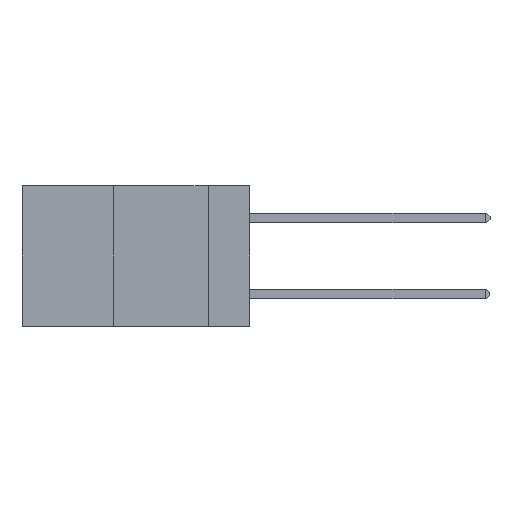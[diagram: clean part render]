
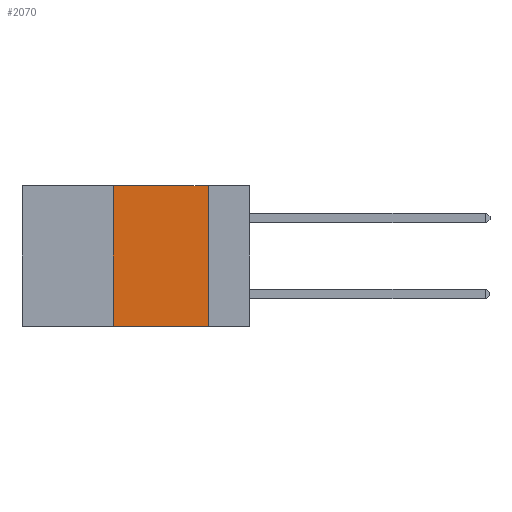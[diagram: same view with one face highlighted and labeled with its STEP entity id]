
A CAD part, left-side view. The second image highlights one B-rep face of the part: STEP entity #2070.
In plain terms, the highlighted planar face has unit normal (-1, 0, 0).
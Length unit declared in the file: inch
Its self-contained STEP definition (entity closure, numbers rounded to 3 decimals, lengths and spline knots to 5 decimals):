
#400 = VERTEX_POINT ( 'NONE', #1898 ) ;
#686 = CARTESIAN_POINT ( 'NONE',  ( 0., 0.36, 0. ) ) ;
#805 = LINE ( 'NONE', #8041, #7409 ) ;
#1435 = DIRECTION ( 'NONE',  ( 1., 0., 0. ) ) ;
#1520 = DIRECTION ( 'NONE',  ( 0., 0., -1. ) ) ;
#1556 = DIRECTION ( 'NONE',  ( 0., 0., 1. ) ) ;
#1810 = LINE ( 'NONE', #4463, #9916 ) ;
#1898 = CARTESIAN_POINT ( 'NONE',  ( 0., 0.36, -0.37 ) ) ;
#1945 = CARTESIAN_POINT ( 'NONE',  ( 0., 0.11, 0. ) ) ;
#2070 = ADVANCED_FACE ( 'NONE', ( #2099 ), #2226, .F. ) ;
#2099 = FACE_OUTER_BOUND ( 'NONE', #4764, .T. ) ;
#2226 = PLANE ( 'NONE',  #4712 ) ;
#2242 = EDGE_CURVE ( 'NONE', #400, #5121, #1810, .T. ) ;
#2275 = EDGE_CURVE ( 'NONE', #4352, #5121, #6073, .T. ) ;
#2373 = ORIENTED_EDGE ( 'NONE', *, *, #9530, .F. ) ;
#3646 = VECTOR ( 'NONE', #1556, 39.37008 ) ;
#3748 = EDGE_CURVE ( 'NONE', #6074, #4352, #805, .T. ) ;
#3892 = VECTOR ( 'NONE', #6697, 39.37008 ) ;
#4128 = DIRECTION ( 'NONE',  ( 0., -1., 0. ) ) ;
#4352 = VERTEX_POINT ( 'NONE', #9914 ) ;
#4375 = ORIENTED_EDGE ( 'NONE', *, *, #2275, .F. ) ;
#4463 = CARTESIAN_POINT ( 'NONE',  ( 0., 0.6, -0.37 ) ) ;
#4712 = AXIS2_PLACEMENT_3D ( 'NONE', #7211, #1435, #1520 ) ;
#4764 = EDGE_LOOP ( 'NONE', ( #4375, #6512, #2373, #6731 ) ) ;
#5121 = VERTEX_POINT ( 'NONE', #8416 ) ;
#5589 = LINE ( 'NONE', #686, #3646 ) ;
#6073 = LINE ( 'NONE', #1945, #3892 ) ;
#6074 = VERTEX_POINT ( 'NONE', #9123 ) ;
#6512 = ORIENTED_EDGE ( 'NONE', *, *, #3748, .F. ) ;
#6697 = DIRECTION ( 'NONE',  ( 0., 0., -1. ) ) ;
#6731 = ORIENTED_EDGE ( 'NONE', *, *, #2242, .T. ) ;
#7211 = CARTESIAN_POINT ( 'NONE',  ( 0., 0.6, 0. ) ) ;
#7409 = VECTOR ( 'NONE', #7955, 39.37008 ) ;
#7955 = DIRECTION ( 'NONE',  ( 0., -1., 0. ) ) ;
#8041 = CARTESIAN_POINT ( 'NONE',  ( 0., 0.6, 0. ) ) ;
#8416 = CARTESIAN_POINT ( 'NONE',  ( 0., 0.11, -0.37 ) ) ;
#9123 = CARTESIAN_POINT ( 'NONE',  ( 0., 0.36, 0. ) ) ;
#9530 = EDGE_CURVE ( 'NONE', #400, #6074, #5589, .T. ) ;
#9914 = CARTESIAN_POINT ( 'NONE',  ( 0., 0.11, 0. ) ) ;
#9916 = VECTOR ( 'NONE', #4128, 39.37008 ) ;
